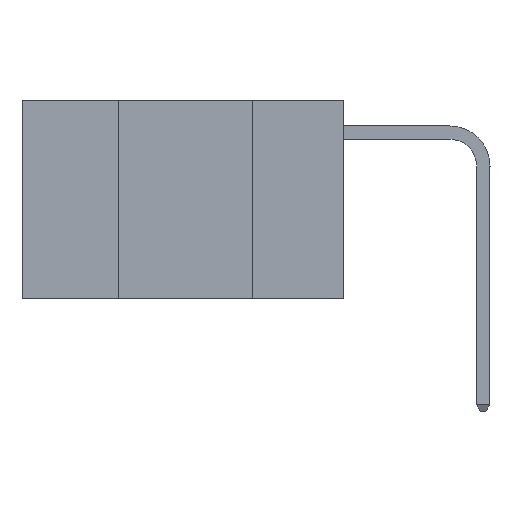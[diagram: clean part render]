
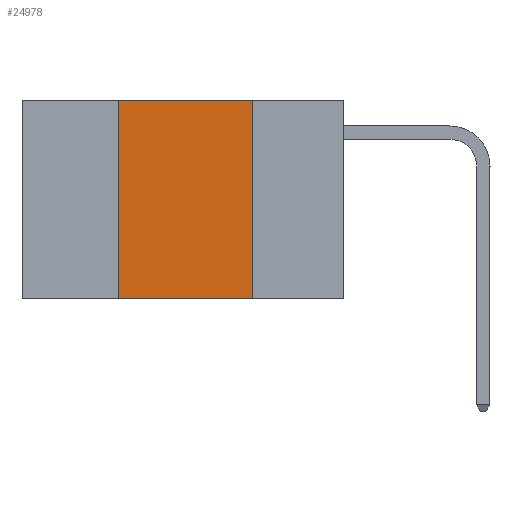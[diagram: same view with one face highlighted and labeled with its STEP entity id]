
A CAD part, left-side view. The second image highlights one B-rep face of the part: STEP entity #24978.
In plain terms, the highlighted planar face has unit normal (-1, 0, 0).
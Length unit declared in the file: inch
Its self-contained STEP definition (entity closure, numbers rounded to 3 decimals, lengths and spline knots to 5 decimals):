
#69 = VECTOR ( 'NONE', #22270, 39.37008 ) ;
#557 = ORIENTED_EDGE ( 'NONE', *, *, #12756, .F. ) ;
#799 = DIRECTION ( 'NONE',  ( 0., -1., 0. ) ) ;
#1409 = CARTESIAN_POINT ( 'NONE',  ( 0., 0.17, 0. ) ) ;
#1877 = CARTESIAN_POINT ( 'NONE',  ( 0., 0.42, -0.37 ) ) ;
#4322 = EDGE_CURVE ( 'NONE', #13067, #15725, #17741, .T. ) ;
#4649 = EDGE_CURVE ( 'NONE', #13067, #18161, #15433, .T. ) ;
#4833 = CARTESIAN_POINT ( 'NONE',  ( 0., 0.17, 0. ) ) ;
#6356 = EDGE_CURVE ( 'NONE', #9251, #15725, #16679, .T. ) ;
#6668 = VECTOR ( 'NONE', #20636, 39.37008 ) ;
#9218 = DIRECTION ( 'NONE',  ( 1., 0., 0. ) ) ;
#9251 = VERTEX_POINT ( 'NONE', #4833 ) ;
#9339 = FACE_OUTER_BOUND ( 'NONE', #24172, .T. ) ;
#10877 = AXIS2_PLACEMENT_3D ( 'NONE', #21760, #9218, #23851 ) ;
#11065 = CARTESIAN_POINT ( 'NONE',  ( 0., 0.6, 0. ) ) ;
#12756 = EDGE_CURVE ( 'NONE', #18161, #9251, #12909, .T. ) ;
#12909 = LINE ( 'NONE', #11065, #23382 ) ;
#13067 = VERTEX_POINT ( 'NONE', #1877 ) ;
#14304 = CARTESIAN_POINT ( 'NONE',  ( 0., 0.6, -0.37 ) ) ;
#15433 = LINE ( 'NONE', #19594, #20367 ) ;
#15725 = VERTEX_POINT ( 'NONE', #23952 ) ;
#15840 = ORIENTED_EDGE ( 'NONE', *, *, #6356, .F. ) ;
#16679 = LINE ( 'NONE', #1409, #69 ) ;
#17154 = ORIENTED_EDGE ( 'NONE', *, *, #4649, .F. ) ;
#17741 = LINE ( 'NONE', #14304, #6668 ) ;
#18161 = VERTEX_POINT ( 'NONE', #23749 ) ;
#19594 = CARTESIAN_POINT ( 'NONE',  ( 0., 0.42, 0. ) ) ;
#19651 = PLANE ( 'NONE',  #10877 ) ;
#20367 = VECTOR ( 'NONE', #25891, 39.37008 ) ;
#20636 = DIRECTION ( 'NONE',  ( 0., -1., 0. ) ) ;
#21760 = CARTESIAN_POINT ( 'NONE',  ( 0., 0.6, 0. ) ) ;
#22270 = DIRECTION ( 'NONE',  ( 0., 0., -1. ) ) ;
#23382 = VECTOR ( 'NONE', #799, 39.37008 ) ;
#23749 = CARTESIAN_POINT ( 'NONE',  ( 0., 0.42, 0. ) ) ;
#23851 = DIRECTION ( 'NONE',  ( 0., 0., -1. ) ) ;
#23952 = CARTESIAN_POINT ( 'NONE',  ( 0., 0.17, -0.37 ) ) ;
#24024 = ORIENTED_EDGE ( 'NONE', *, *, #4322, .T. ) ;
#24172 = EDGE_LOOP ( 'NONE', ( #15840, #557, #17154, #24024 ) ) ;
#24978 = ADVANCED_FACE ( 'NONE', ( #9339 ), #19651, .F. ) ;
#25891 = DIRECTION ( 'NONE',  ( 0., 0., 1. ) ) ;
